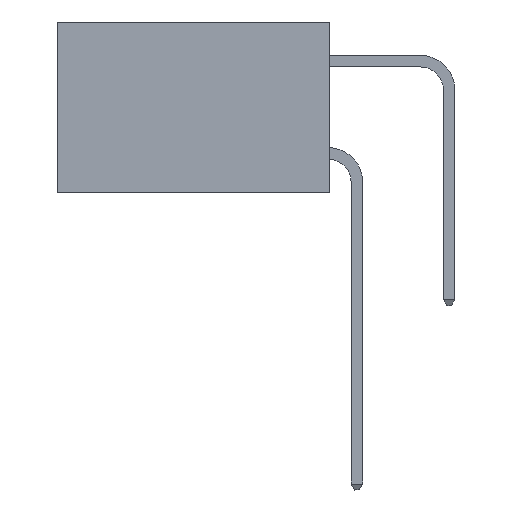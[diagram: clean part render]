
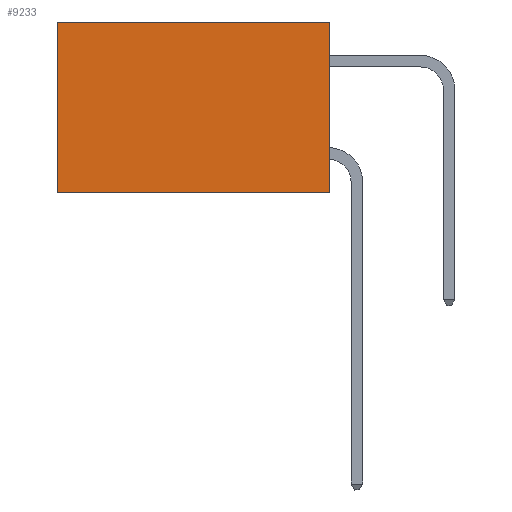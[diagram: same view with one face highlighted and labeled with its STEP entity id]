
A CAD part, left-side view. The second image highlights one B-rep face of the part: STEP entity #9233.
In plain terms, the highlighted planar face has unit normal (-1, 0, 0).
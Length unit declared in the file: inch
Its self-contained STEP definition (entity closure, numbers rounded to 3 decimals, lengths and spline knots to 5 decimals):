
#20 = VECTOR ( 'NONE', #7230, 39.37008 ) ;
#35 = PLANE ( 'NONE',  #3113 ) ;
#93 = CARTESIAN_POINT ( 'NONE',  ( 0.277, 0., -0.37 ) ) ;
#1459 = DIRECTION ( 'NONE',  ( 0., 0., -1. ) ) ;
#2326 = FACE_OUTER_BOUND ( 'NONE', #14188, .T. ) ;
#2416 = EDGE_CURVE ( 'NONE', #12452, #4875, #15878, .T. ) ;
#3113 = AXIS2_PLACEMENT_3D ( 'NONE', #93, #9264, #1459 ) ;
#4002 = CARTESIAN_POINT ( 'NONE',  ( 0.277, 0.59, -0.37 ) ) ;
#4672 = EDGE_CURVE ( 'NONE', #12452, #8933, #7412, .T. ) ;
#4875 = VERTEX_POINT ( 'NONE', #5469 ) ;
#5469 = CARTESIAN_POINT ( 'NONE',  ( 0.277, 0.59, 0. ) ) ;
#5728 = VECTOR ( 'NONE', #9802, 39.37008 ) ;
#5802 = ORIENTED_EDGE ( 'NONE', *, *, #2416, .T. ) ;
#6690 = VECTOR ( 'NONE', #9171, 39.37008 ) ;
#6710 = VECTOR ( 'NONE', #16306, 39.37008 ) ;
#7220 = ORIENTED_EDGE ( 'NONE', *, *, #13068, .T. ) ;
#7230 = DIRECTION ( 'NONE',  ( 0., 0., -1. ) ) ;
#7281 = CARTESIAN_POINT ( 'NONE',  ( 0.277, 0., -0.37 ) ) ;
#7388 = CARTESIAN_POINT ( 'NONE',  ( 0.277, 0., -0.37 ) ) ;
#7412 = LINE ( 'NONE', #7281, #20 ) ;
#8325 = CARTESIAN_POINT ( 'NONE',  ( 0.277, 0., -0.37 ) ) ;
#8445 = ORIENTED_EDGE ( 'NONE', *, *, #12603, .F. ) ;
#8933 = VERTEX_POINT ( 'NONE', #7388 ) ;
#9171 = DIRECTION ( 'NONE',  ( 0., 0., -1. ) ) ;
#9233 = ADVANCED_FACE ( 'NONE', ( #2326 ), #35, .F. ) ;
#9264 = DIRECTION ( 'NONE',  ( 1., 0., 0. ) ) ;
#9350 = CARTESIAN_POINT ( 'NONE',  ( 0.277, 0., 0. ) ) ;
#9442 = CARTESIAN_POINT ( 'NONE',  ( 0.277, 0., 0. ) ) ;
#9802 = DIRECTION ( 'NONE',  ( 0., 1., 0. ) ) ;
#12188 = VERTEX_POINT ( 'NONE', #16773 ) ;
#12452 = VERTEX_POINT ( 'NONE', #9350 ) ;
#12603 = EDGE_CURVE ( 'NONE', #8933, #12188, #13737, .T. ) ;
#13068 = EDGE_CURVE ( 'NONE', #4875, #12188, #13299, .T. ) ;
#13299 = LINE ( 'NONE', #4002, #6690 ) ;
#13737 = LINE ( 'NONE', #8325, #6710 ) ;
#14188 = EDGE_LOOP ( 'NONE', ( #7220, #8445, #15962, #5802 ) ) ;
#15878 = LINE ( 'NONE', #9442, #5728 ) ;
#15962 = ORIENTED_EDGE ( 'NONE', *, *, #4672, .F. ) ;
#16306 = DIRECTION ( 'NONE',  ( 0., 1., 0. ) ) ;
#16773 = CARTESIAN_POINT ( 'NONE',  ( 0.277, 0.59, -0.37 ) ) ;
